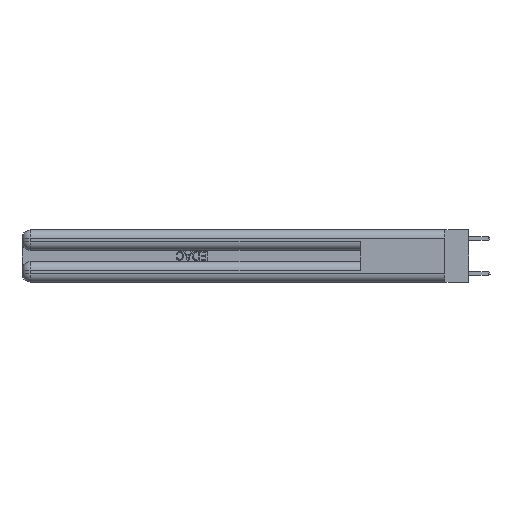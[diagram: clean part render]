
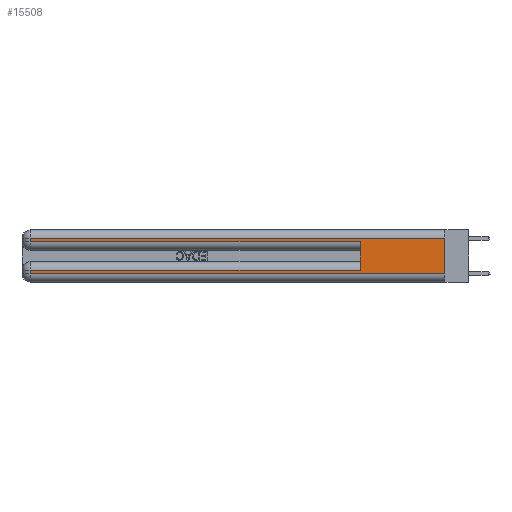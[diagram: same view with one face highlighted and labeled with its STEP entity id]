
A CAD part, left-side view. The second image highlights one B-rep face of the part: STEP entity #15508.
In plain terms, the highlighted planar face has unit normal (-1, 0, 0).
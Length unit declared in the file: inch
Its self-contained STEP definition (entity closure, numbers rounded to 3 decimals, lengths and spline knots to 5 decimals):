
#310 = VERTEX_POINT ( 'NONE', #1844 ) ;
#569 = VECTOR ( 'NONE', #24142, 39.37008 ) ;
#1016 = PLANE ( 'NONE',  #3541 ) ;
#1021 = EDGE_CURVE ( 'NONE', #4450, #310, #12467, .T. ) ;
#1844 = CARTESIAN_POINT ( 'NONE',  ( 0., 2.94, 0.085 ) ) ;
#2504 = DIRECTION ( 'NONE',  ( 0., 0., -1. ) ) ;
#3108 = CARTESIAN_POINT ( 'NONE',  ( 0., 0., 0.37 ) ) ;
#3137 = VECTOR ( 'NONE', #9220, 39.37008 ) ;
#3541 = AXIS2_PLACEMENT_3D ( 'NONE', #3108, #25073, #10799 ) ;
#4420 = LINE ( 'NONE', #6826, #569 ) ;
#4450 = VERTEX_POINT ( 'NONE', #26796 ) ;
#5335 = EDGE_CURVE ( 'NONE', #31169, #8088, #6552, .T. ) ;
#5500 = VECTOR ( 'NONE', #15332, 39.37008 ) ;
#5894 = ORIENTED_EDGE ( 'NONE', *, *, #19788, .T. ) ;
#6552 = LINE ( 'NONE', #25936, #12006 ) ;
#6826 = CARTESIAN_POINT ( 'NONE',  ( 0., 0., 0.06 ) ) ;
#6990 = CARTESIAN_POINT ( 'NONE',  ( 0., 2.94, 0.37 ) ) ;
#7182 = CARTESIAN_POINT ( 'NONE',  ( 0., 0., 0.085 ) ) ;
#7271 = CARTESIAN_POINT ( 'NONE',  ( 0., 2.94, 0.285 ) ) ;
#8064 = CARTESIAN_POINT ( 'NONE',  ( 0., 2.94, 0.31 ) ) ;
#8088 = VERTEX_POINT ( 'NONE', #8064 ) ;
#8469 = LINE ( 'NONE', #6990, #3137 ) ;
#8592 = VERTEX_POINT ( 'NONE', #7271 ) ;
#9220 = DIRECTION ( 'NONE',  ( 0., 0., -1. ) ) ;
#10799 = DIRECTION ( 'NONE',  ( 0., 0., -1. ) ) ;
#11520 = DIRECTION ( 'NONE',  ( 0., 1., 0. ) ) ;
#11856 = VERTEX_POINT ( 'NONE', #11868 ) ;
#11868 = CARTESIAN_POINT ( 'NONE',  ( 0., 2.94, 0.06 ) ) ;
#12006 = VECTOR ( 'NONE', #11520, 39.37008 ) ;
#12275 = VECTOR ( 'NONE', #17397, 39.37008 ) ;
#12464 = EDGE_CURVE ( 'NONE', #8592, #14956, #17740, .T. ) ;
#12467 = LINE ( 'NONE', #7182, #19283 ) ;
#12586 = ORIENTED_EDGE ( 'NONE', *, *, #21260, .F. ) ;
#12948 = ORIENTED_EDGE ( 'NONE', *, *, #1021, .T. ) ;
#14956 = VERTEX_POINT ( 'NONE', #15379 ) ;
#15332 = DIRECTION ( 'NONE',  ( 0., -1., 0. ) ) ;
#15333 = EDGE_CURVE ( 'NONE', #8088, #8592, #21287, .T. ) ;
#15379 = CARTESIAN_POINT ( 'NONE',  ( 0., 0.6, 0.285 ) ) ;
#15508 = ADVANCED_FACE ( 'NONE', ( #25224 ), #1016, .F. ) ;
#16903 = CARTESIAN_POINT ( 'NONE',  ( 0., 0.6, 0.145 ) ) ;
#17221 = LINE ( 'NONE', #16903, #25740 ) ;
#17369 = ORIENTED_EDGE ( 'NONE', *, *, #5335, .T. ) ;
#17397 = DIRECTION ( 'NONE',  ( 0., 0., -1. ) ) ;
#17468 = CARTESIAN_POINT ( 'NONE',  ( 0., 0., 0.06 ) ) ;
#17740 = LINE ( 'NONE', #27497, #5500 ) ;
#17921 = ORIENTED_EDGE ( 'NONE', *, *, #19859, .T. ) ;
#18591 = LINE ( 'NONE', #25950, #23176 ) ;
#19283 = VECTOR ( 'NONE', #22084, 39.37008 ) ;
#19788 = EDGE_CURVE ( 'NONE', #310, #11856, #8469, .T. ) ;
#19859 = EDGE_CURVE ( 'NONE', #11856, #27035, #4420, .T. ) ;
#20339 = CARTESIAN_POINT ( 'NONE',  ( 0., 0., 0.31 ) ) ;
#21260 = EDGE_CURVE ( 'NONE', #31169, #27035, #18591, .T. ) ;
#21287 = LINE ( 'NONE', #31037, #12275 ) ;
#21620 = ORIENTED_EDGE ( 'NONE', *, *, #12464, .T. ) ;
#21691 = EDGE_CURVE ( 'NONE', #4450, #14956, #17221, .T. ) ;
#22084 = DIRECTION ( 'NONE',  ( 0., 1., 0. ) ) ;
#22092 = ORIENTED_EDGE ( 'NONE', *, *, #21691, .F. ) ;
#23176 = VECTOR ( 'NONE', #2504, 39.37008 ) ;
#23295 = EDGE_LOOP ( 'NONE', ( #12586, #17369, #28113, #21620, #22092, #12948, #5894, #17921 ) ) ;
#24142 = DIRECTION ( 'NONE',  ( 0., -1., 0. ) ) ;
#25073 = DIRECTION ( 'NONE',  ( 1., 0., 0. ) ) ;
#25224 = FACE_OUTER_BOUND ( 'NONE', #23295, .T. ) ;
#25740 = VECTOR ( 'NONE', #26815, 39.37008 ) ;
#25936 = CARTESIAN_POINT ( 'NONE',  ( 0., 0., 0.31 ) ) ;
#25950 = CARTESIAN_POINT ( 'NONE',  ( 0., 0., 0.37 ) ) ;
#26796 = CARTESIAN_POINT ( 'NONE',  ( 0., 0.6, 0.085 ) ) ;
#26815 = DIRECTION ( 'NONE',  ( 0., 0., 1. ) ) ;
#27035 = VERTEX_POINT ( 'NONE', #17468 ) ;
#27497 = CARTESIAN_POINT ( 'NONE',  ( 0., 0., 0.285 ) ) ;
#28113 = ORIENTED_EDGE ( 'NONE', *, *, #15333, .T. ) ;
#31037 = CARTESIAN_POINT ( 'NONE',  ( 0., 2.94, 0.37 ) ) ;
#31169 = VERTEX_POINT ( 'NONE', #20339 ) ;
